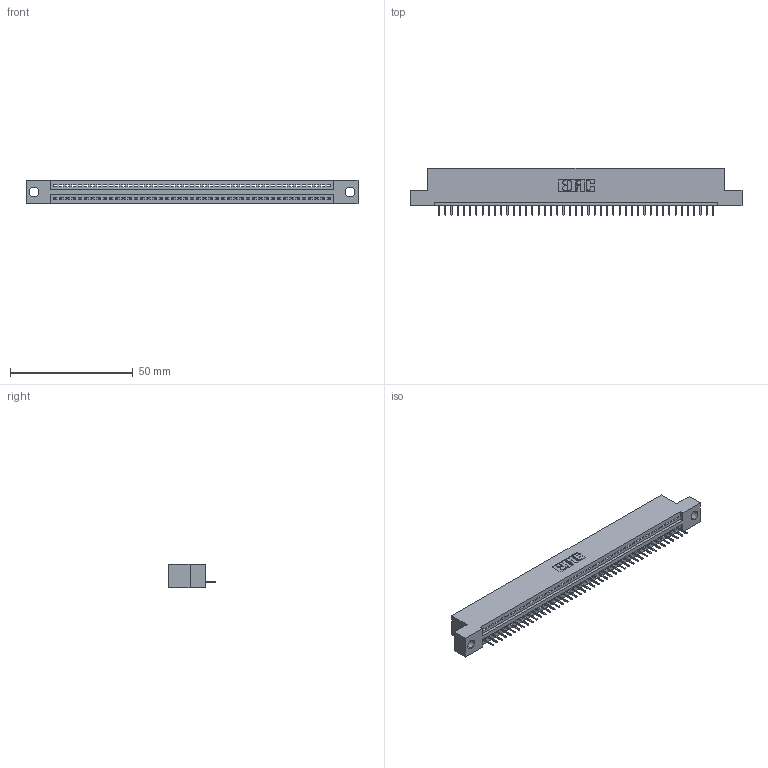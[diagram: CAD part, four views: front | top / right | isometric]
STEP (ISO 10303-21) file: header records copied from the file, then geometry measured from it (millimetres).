
FILE_DESCRIPTION (( 'STEP AP203' ), '1' );
FILE_NAME ('395-045-524-104.STEP', '2021-05-31T15:10:43', ( '' ), ( '' ), 'SwSTEP 2.0', 'SolidWorks 2020', '' );
FILE_SCHEMA (( 'CONFIG_CONTROL_DESIGN' ));
Length unit declared in the file: inch
Products named in the file (3): 395-045-524-104; 345 Part_Flush Mounting Lugs - 0.156 Dia-TI; 345-292-001_345-293-124
Assembly tree (46 placements, depth 2):
  395-045-524-104
    345 Part_Flush Mounting Lugs - 0.156 Dia-TI
    345-292-001_345-293-124  x45
Bounding box: 135.51 x 19.35 x 9.4 mm (x, y, z)
Volume: 12611.6 mm3; surface area: 16074.6 mm2
Topology: 46 solids, 46 shells, 2930 faces, 8477 edges, 5470 vertices
Faces by surface type: plane 2164, cylinder 766
Entity records: 33957 total; most frequent: CARTESIAN_POINT 5889, ORIENTED_EDGE 5866, DIRECTION 5139, EDGE_CURVE 2933, VECTOR 2625, LINE 2625, VERTEX_POINT 1950, AXIS2_PLACEMENT_3D 1257
